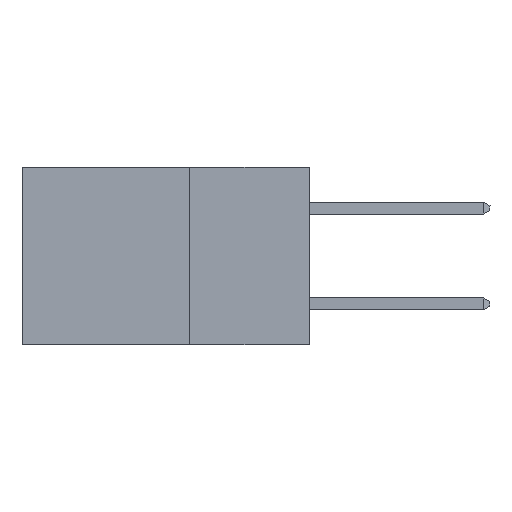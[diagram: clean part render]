
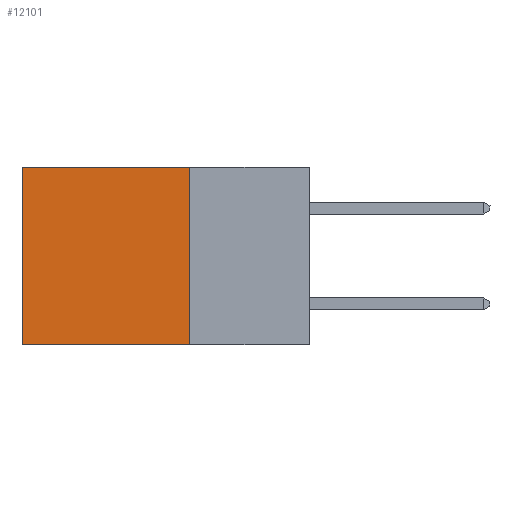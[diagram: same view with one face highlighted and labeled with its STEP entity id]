
A CAD part, left-side view. The second image highlights one B-rep face of the part: STEP entity #12101.
In plain terms, the highlighted planar face has unit normal (-1, 0, 0).
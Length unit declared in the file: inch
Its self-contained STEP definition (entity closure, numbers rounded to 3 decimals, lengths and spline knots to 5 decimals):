
#530 = ORIENTED_EDGE ( 'NONE', *, *, #2618, .T. ) ;
#583 = ORIENTED_EDGE ( 'NONE', *, *, #4295, .F. ) ;
#765 = ORIENTED_EDGE ( 'NONE', *, *, #2847, .F. ) ;
#917 = ORIENTED_EDGE ( 'NONE', *, *, #5553, .T. ) ;
#1204 = PLANE ( 'NONE',  #1543 ) ;
#1543 = AXIS2_PLACEMENT_3D ( 'NONE', #9035, #9088, #2345 ) ;
#1976 = VECTOR ( 'NONE', #7215, 39.37008 ) ;
#2005 = CARTESIAN_POINT ( 'NONE',  ( 0.2875, 0.25, -0.37 ) ) ;
#2345 = DIRECTION ( 'NONE',  ( 0., 0., -1. ) ) ;
#2437 = VECTOR ( 'NONE', #13026, 39.37008 ) ;
#2512 = VECTOR ( 'NONE', #4682, 39.37008 ) ;
#2618 = EDGE_CURVE ( 'NONE', #3566, #4484, #5685, .T. ) ;
#2830 = CARTESIAN_POINT ( 'NONE',  ( 0.2875, 0.25, -0.37 ) ) ;
#2847 = EDGE_CURVE ( 'NONE', #7732, #3757, #8465, .T. ) ;
#3566 = VERTEX_POINT ( 'NONE', #7746 ) ;
#3757 = VERTEX_POINT ( 'NONE', #2005 ) ;
#4295 = EDGE_CURVE ( 'NONE', #3757, #4484, #11132, .T. ) ;
#4484 = VERTEX_POINT ( 'NONE', #12266 ) ;
#4682 = DIRECTION ( 'NONE',  ( 0., 0., -1. ) ) ;
#5039 = CARTESIAN_POINT ( 'NONE',  ( 0.2875, 0.25, 0. ) ) ;
#5553 = EDGE_CURVE ( 'NONE', #7732, #3566, #8409, .T. ) ;
#5685 = LINE ( 'NONE', #7316, #1976 ) ;
#7215 = DIRECTION ( 'NONE',  ( 0., 0., -1. ) ) ;
#7316 = CARTESIAN_POINT ( 'NONE',  ( 0.2875, 0.6, 0. ) ) ;
#7732 = VERTEX_POINT ( 'NONE', #10024 ) ;
#7746 = CARTESIAN_POINT ( 'NONE',  ( 0.2875, 0.6, 0. ) ) ;
#7876 = CARTESIAN_POINT ( 'NONE',  ( 0.2875, 0.25, 0. ) ) ;
#8409 = LINE ( 'NONE', #7876, #2437 ) ;
#8465 = LINE ( 'NONE', #5039, #2512 ) ;
#9035 = CARTESIAN_POINT ( 'NONE',  ( 0.2875, 0.25, 0. ) ) ;
#9088 = DIRECTION ( 'NONE',  ( 1., 0., 0. ) ) ;
#10024 = CARTESIAN_POINT ( 'NONE',  ( 0.2875, 0.25, 0. ) ) ;
#10108 = FACE_OUTER_BOUND ( 'NONE', #11826, .T. ) ;
#10495 = VECTOR ( 'NONE', #12180, 39.37008 ) ;
#11132 = LINE ( 'NONE', #2830, #10495 ) ;
#11826 = EDGE_LOOP ( 'NONE', ( #530, #583, #765, #917 ) ) ;
#12101 = ADVANCED_FACE ( 'NONE', ( #10108 ), #1204, .F. ) ;
#12180 = DIRECTION ( 'NONE',  ( 0., 1., 0. ) ) ;
#12266 = CARTESIAN_POINT ( 'NONE',  ( 0.2875, 0.6, -0.37 ) ) ;
#13026 = DIRECTION ( 'NONE',  ( 0., 1., 0. ) ) ;
